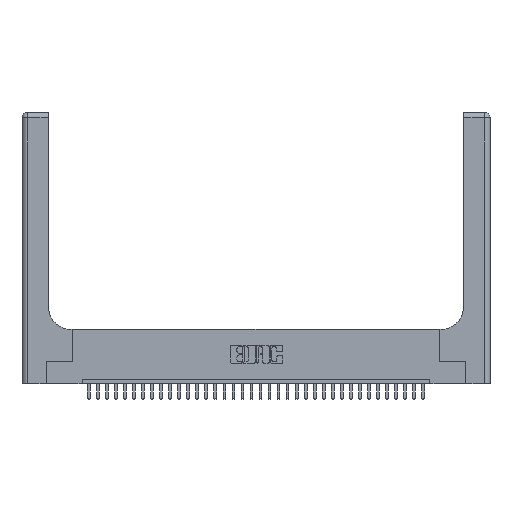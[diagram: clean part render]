
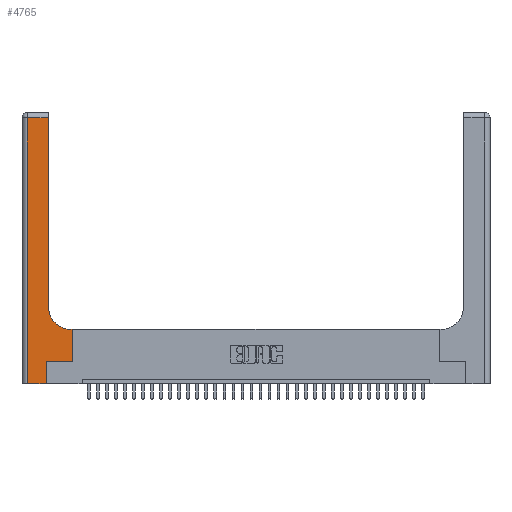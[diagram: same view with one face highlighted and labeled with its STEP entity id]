
A CAD part, top view. The second image highlights one B-rep face of the part: STEP entity #4765.
In plain terms, the highlighted planar face has unit normal (0, 0, 1).
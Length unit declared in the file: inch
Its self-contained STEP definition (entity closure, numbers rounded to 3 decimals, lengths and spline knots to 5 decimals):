
#219 = VERTEX_POINT ( 'NONE', #5494 ) ;
#278 = ORIENTED_EDGE ( 'NONE', *, *, #11777, .T. ) ;
#440 = ORIENTED_EDGE ( 'NONE', *, *, #27817, .T. ) ;
#1015 = VECTOR ( 'NONE', #10341, 39.37008 ) ;
#1103 = DIRECTION ( 'NONE',  ( 0., 0., -1. ) ) ;
#2030 = DIRECTION ( 'NONE',  ( -1., 0., 0. ) ) ;
#2128 = LINE ( 'NONE', #21830, #32091 ) ;
#2248 = EDGE_CURVE ( 'NONE', #24327, #22380, #2128, .T. ) ;
#2362 = LINE ( 'NONE', #4641, #22711 ) ;
#2435 = CARTESIAN_POINT ( 'NONE',  ( 0.269, 0., 0.37 ) ) ;
#3764 = CARTESIAN_POINT ( 'NONE',  ( 0., 3., 0.37 ) ) ;
#4641 = CARTESIAN_POINT ( 'NONE',  ( 0., 2.94, 0.37 ) ) ;
#4765 = ADVANCED_FACE ( 'NONE', ( #9693 ), #11522, .F. ) ;
#5223 = LINE ( 'NONE', #14039, #13103 ) ;
#5290 = EDGE_LOOP ( 'NONE', ( #8397, #9722, #440, #278, #12812, #9605, #13299, #20533, #13535 ) ) ;
#5494 = CARTESIAN_POINT ( 'NONE',  ( 0.5415, 0.6, 0.37 ) ) ;
#6514 = AXIS2_PLACEMENT_3D ( 'NONE', #7070, #25945, #10027 ) ;
#7070 = CARTESIAN_POINT ( 'NONE',  ( 0.5415, 0.85, 0.37 ) ) ;
#7521 = VECTOR ( 'NONE', #2030, 39.37008 ) ;
#7821 = CARTESIAN_POINT ( 'NONE',  ( 0., 0., 0.37 ) ) ;
#8312 = VECTOR ( 'NONE', #22972, 39.37008 ) ;
#8397 = ORIENTED_EDGE ( 'NONE', *, *, #30864, .T. ) ;
#9339 = LINE ( 'NONE', #2435, #1015 ) ;
#9605 = ORIENTED_EDGE ( 'NONE', *, *, #24096, .T. ) ;
#9693 = FACE_OUTER_BOUND ( 'NONE', #5290, .T. ) ;
#9722 = ORIENTED_EDGE ( 'NONE', *, *, #13124, .T. ) ;
#9940 = DIRECTION ( 'NONE',  ( -1., 0., 0. ) ) ;
#10027 = DIRECTION ( 'NONE',  ( 1., 0., 0. ) ) ;
#10341 = DIRECTION ( 'NONE',  ( 0., 1., 0. ) ) ;
#11254 = EDGE_CURVE ( 'NONE', #22380, #219, #32462, .T. ) ;
#11265 = DIRECTION ( 'NONE',  ( 0., 1., 0. ) ) ;
#11522 = PLANE ( 'NONE',  #16106 ) ;
#11777 = EDGE_CURVE ( 'NONE', #34272, #32777, #31164, .T. ) ;
#12004 = VECTOR ( 'NONE', #11265, 39.37008 ) ;
#12080 = CARTESIAN_POINT ( 'NONE',  ( 0.269, 0.25, 0.37 ) ) ;
#12812 = ORIENTED_EDGE ( 'NONE', *, *, #32959, .T. ) ;
#13103 = VECTOR ( 'NONE', #19264, 39.37008 ) ;
#13124 = EDGE_CURVE ( 'NONE', #29026, #21806, #2362, .T. ) ;
#13299 = ORIENTED_EDGE ( 'NONE', *, *, #2248, .T. ) ;
#13535 = ORIENTED_EDGE ( 'NONE', *, *, #21993, .T. ) ;
#14033 = CARTESIAN_POINT ( 'NONE',  ( 0.2915, 3., 0.37 ) ) ;
#14039 = CARTESIAN_POINT ( 'NONE',  ( 0.269, 0.25, 0.37 ) ) ;
#14171 = DIRECTION ( 'NONE',  ( -1., 0., 0. ) ) ;
#14279 = VERTEX_POINT ( 'NONE', #12080 ) ;
#14931 = CARTESIAN_POINT ( 'NONE',  ( 0.06, 3., 0.37 ) ) ;
#15346 = CARTESIAN_POINT ( 'NONE',  ( 0.2915, 0.6, 0.37 ) ) ;
#16106 = AXIS2_PLACEMENT_3D ( 'NONE', #3764, #1103, #14171 ) ;
#16524 = LINE ( 'NONE', #14033, #12004 ) ;
#16874 = CIRCLE ( 'NONE', #6514, 0.25 ) ;
#16876 = CARTESIAN_POINT ( 'NONE',  ( 0.2915, 0.85, 0.37 ) ) ;
#19264 = DIRECTION ( 'NONE',  ( 1., 0., 0. ) ) ;
#19486 = CARTESIAN_POINT ( 'NONE',  ( 0.5585, 0.6, 0.37 ) ) ;
#20533 = ORIENTED_EDGE ( 'NONE', *, *, #11254, .T. ) ;
#21716 = DIRECTION ( 'NONE',  ( 0., 1., 0. ) ) ;
#21806 = VERTEX_POINT ( 'NONE', #33209 ) ;
#21830 = CARTESIAN_POINT ( 'NONE',  ( 0.5585, 0.25, 0.37 ) ) ;
#21993 = EDGE_CURVE ( 'NONE', #219, #33116, #16874, .T. ) ;
#22380 = VERTEX_POINT ( 'NONE', #19486 ) ;
#22711 = VECTOR ( 'NONE', #9940, 39.37008 ) ;
#22972 = DIRECTION ( 'NONE',  ( 0., -1., 0. ) ) ;
#23232 = VECTOR ( 'NONE', #23939, 39.37008 ) ;
#23939 = DIRECTION ( 'NONE',  ( 1., 0., 0. ) ) ;
#24096 = EDGE_CURVE ( 'NONE', #14279, #24327, #5223, .T. ) ;
#24327 = VERTEX_POINT ( 'NONE', #28491 ) ;
#25811 = CARTESIAN_POINT ( 'NONE',  ( 0.2915, 2.94, 0.37 ) ) ;
#25945 = DIRECTION ( 'NONE',  ( 0., 0., -1. ) ) ;
#27412 = CARTESIAN_POINT ( 'NONE',  ( 0.06, 0., 0.37 ) ) ;
#27800 = CARTESIAN_POINT ( 'NONE',  ( 0.269, 0., 0.37 ) ) ;
#27817 = EDGE_CURVE ( 'NONE', #21806, #34272, #30404, .T. ) ;
#28491 = CARTESIAN_POINT ( 'NONE',  ( 0.5585, 0.25, 0.37 ) ) ;
#29026 = VERTEX_POINT ( 'NONE', #25811 ) ;
#30404 = LINE ( 'NONE', #14931, #8312 ) ;
#30864 = EDGE_CURVE ( 'NONE', #33116, #29026, #16524, .T. ) ;
#31164 = LINE ( 'NONE', #7821, #23232 ) ;
#32091 = VECTOR ( 'NONE', #21716, 39.37008 ) ;
#32462 = LINE ( 'NONE', #15346, #7521 ) ;
#32777 = VERTEX_POINT ( 'NONE', #27800 ) ;
#32959 = EDGE_CURVE ( 'NONE', #32777, #14279, #9339, .T. ) ;
#33116 = VERTEX_POINT ( 'NONE', #16876 ) ;
#33209 = CARTESIAN_POINT ( 'NONE',  ( 0.06, 2.94, 0.37 ) ) ;
#34272 = VERTEX_POINT ( 'NONE', #27412 ) ;
